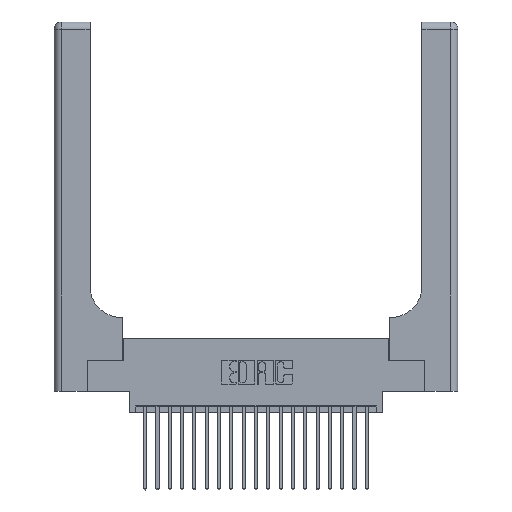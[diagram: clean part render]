
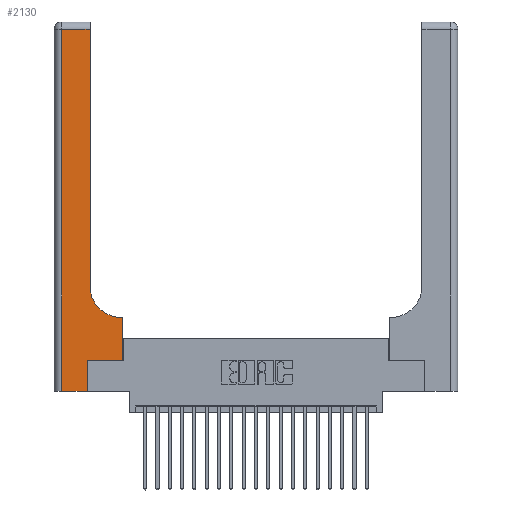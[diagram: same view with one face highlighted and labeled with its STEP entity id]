
A CAD part, top view. The second image highlights one B-rep face of the part: STEP entity #2130.
In plain terms, the highlighted planar face has unit normal (0, 0, 1).
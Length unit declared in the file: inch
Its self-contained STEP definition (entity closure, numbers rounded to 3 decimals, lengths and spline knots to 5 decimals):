
#53 = LINE ( 'NONE', #11042, #6260 ) ;
#124 = ORIENTED_EDGE ( 'NONE', *, *, #6037, .T. ) ;
#2130 = ADVANCED_FACE ( 'NONE', ( #3222 ), #7869, .F. ) ;
#2428 = CARTESIAN_POINT ( 'NONE',  ( 0.269, 0., 0.37 ) ) ;
#2533 = DIRECTION ( 'NONE',  ( 0., 1., 0. ) ) ;
#2838 = EDGE_CURVE ( 'NONE', #14635, #17564, #6567, .T. ) ;
#3041 = CARTESIAN_POINT ( 'NONE',  ( 0.2915, 2.94, 0.37 ) ) ;
#3222 = FACE_OUTER_BOUND ( 'NONE', #5168, .T. ) ;
#3240 = CARTESIAN_POINT ( 'NONE',  ( 0.5585, 0.6, 0.37 ) ) ;
#3610 = AXIS2_PLACEMENT_3D ( 'NONE', #22435, #18960, #9760 ) ;
#4434 = DIRECTION ( 'NONE',  ( 0., 1., 0. ) ) ;
#4953 = VECTOR ( 'NONE', #19559, 39.37008 ) ;
#5168 = EDGE_LOOP ( 'NONE', ( #18181, #15463, #124, #20148, #8820, #6067, #8942, #13256, #19087 ) ) ;
#5347 = EDGE_CURVE ( 'NONE', #8840, #13324, #22948, .T. ) ;
#5991 = VECTOR ( 'NONE', #2533, 39.37008 ) ;
#6037 = EDGE_CURVE ( 'NONE', #12540, #9244, #12771, .T. ) ;
#6067 = ORIENTED_EDGE ( 'NONE', *, *, #5347, .T. ) ;
#6260 = VECTOR ( 'NONE', #10792, 39.37008 ) ;
#6567 = LINE ( 'NONE', #13313, #5991 ) ;
#6883 = CARTESIAN_POINT ( 'NONE',  ( 0.5585, 0.25, 0.37 ) ) ;
#6976 = EDGE_CURVE ( 'NONE', #13324, #9922, #53, .T. ) ;
#7041 = CARTESIAN_POINT ( 'NONE',  ( 0.5415, 0.6, 0.37 ) ) ;
#7109 = CARTESIAN_POINT ( 'NONE',  ( 0.5415, 0.85, 0.37 ) ) ;
#7869 = PLANE ( 'NONE',  #3610 ) ;
#8820 = ORIENTED_EDGE ( 'NONE', *, *, #9783, .T. ) ;
#8840 = VERTEX_POINT ( 'NONE', #22633 ) ;
#8942 = ORIENTED_EDGE ( 'NONE', *, *, #6976, .T. ) ;
#9244 = VERTEX_POINT ( 'NONE', #16333 ) ;
#9751 = EDGE_CURVE ( 'NONE', #17564, #12540, #16808, .T. ) ;
#9760 = DIRECTION ( 'NONE',  ( -1., 0., 0. ) ) ;
#9783 = EDGE_CURVE ( 'NONE', #22295, #8840, #10376, .T. ) ;
#9922 = VERTEX_POINT ( 'NONE', #3240 ) ;
#10376 = LINE ( 'NONE', #2428, #17395 ) ;
#10676 = VECTOR ( 'NONE', #15956, 39.37008 ) ;
#10792 = DIRECTION ( 'NONE',  ( 0., 1., 0. ) ) ;
#11042 = CARTESIAN_POINT ( 'NONE',  ( 0.5585, 0.25, 0.37 ) ) ;
#11755 = EDGE_CURVE ( 'NONE', #9922, #15126, #20685, .T. ) ;
#12521 = EDGE_CURVE ( 'NONE', #9244, #22295, #16586, .T. ) ;
#12540 = VERTEX_POINT ( 'NONE', #19642 ) ;
#12771 = LINE ( 'NONE', #16978, #16181 ) ;
#12901 = AXIS2_PLACEMENT_3D ( 'NONE', #7109, #21331, #17549 ) ;
#13256 = ORIENTED_EDGE ( 'NONE', *, *, #11755, .T. ) ;
#13313 = CARTESIAN_POINT ( 'NONE',  ( 0.2915, 3., 0.37 ) ) ;
#13324 = VERTEX_POINT ( 'NONE', #6883 ) ;
#13684 = DIRECTION ( 'NONE',  ( 0., -1., 0. ) ) ;
#14135 = CARTESIAN_POINT ( 'NONE',  ( 0., 0., 0.37 ) ) ;
#14210 = CARTESIAN_POINT ( 'NONE',  ( 0.269, 0.25, 0.37 ) ) ;
#14635 = VERTEX_POINT ( 'NONE', #15863 ) ;
#14746 = VECTOR ( 'NONE', #17815, 39.37008 ) ;
#15126 = VERTEX_POINT ( 'NONE', #7041 ) ;
#15193 = CARTESIAN_POINT ( 'NONE',  ( 0., 2.94, 0.37 ) ) ;
#15463 = ORIENTED_EDGE ( 'NONE', *, *, #9751, .T. ) ;
#15863 = CARTESIAN_POINT ( 'NONE',  ( 0.2915, 0.85, 0.37 ) ) ;
#15952 = CARTESIAN_POINT ( 'NONE',  ( 0.2915, 0.6, 0.37 ) ) ;
#15956 = DIRECTION ( 'NONE',  ( 1., 0., 0. ) ) ;
#16181 = VECTOR ( 'NONE', #13684, 39.37008 ) ;
#16333 = CARTESIAN_POINT ( 'NONE',  ( 0.06, 0., 0.37 ) ) ;
#16586 = LINE ( 'NONE', #14135, #10676 ) ;
#16808 = LINE ( 'NONE', #15193, #22191 ) ;
#16978 = CARTESIAN_POINT ( 'NONE',  ( 0.06, 3., 0.37 ) ) ;
#17051 = EDGE_CURVE ( 'NONE', #15126, #14635, #21470, .T. ) ;
#17395 = VECTOR ( 'NONE', #4434, 39.37008 ) ;
#17549 = DIRECTION ( 'NONE',  ( 1., 0., 0. ) ) ;
#17564 = VERTEX_POINT ( 'NONE', #3041 ) ;
#17815 = DIRECTION ( 'NONE',  ( 1., 0., 0. ) ) ;
#18181 = ORIENTED_EDGE ( 'NONE', *, *, #2838, .T. ) ;
#18960 = DIRECTION ( 'NONE',  ( 0., 0., -1. ) ) ;
#19087 = ORIENTED_EDGE ( 'NONE', *, *, #17051, .T. ) ;
#19559 = DIRECTION ( 'NONE',  ( -1., 0., 0. ) ) ;
#19642 = CARTESIAN_POINT ( 'NONE',  ( 0.06, 2.94, 0.37 ) ) ;
#20148 = ORIENTED_EDGE ( 'NONE', *, *, #12521, .T. ) ;
#20309 = DIRECTION ( 'NONE',  ( -1., 0., 0. ) ) ;
#20685 = LINE ( 'NONE', #15952, #4953 ) ;
#21331 = DIRECTION ( 'NONE',  ( 0., 0., -1. ) ) ;
#21470 = CIRCLE ( 'NONE', #12901, 0.25 ) ;
#22156 = CARTESIAN_POINT ( 'NONE',  ( 0.269, 0., 0.37 ) ) ;
#22191 = VECTOR ( 'NONE', #20309, 39.37008 ) ;
#22295 = VERTEX_POINT ( 'NONE', #22156 ) ;
#22435 = CARTESIAN_POINT ( 'NONE',  ( 0., 3., 0.37 ) ) ;
#22633 = CARTESIAN_POINT ( 'NONE',  ( 0.269, 0.25, 0.37 ) ) ;
#22948 = LINE ( 'NONE', #14210, #14746 ) ;
